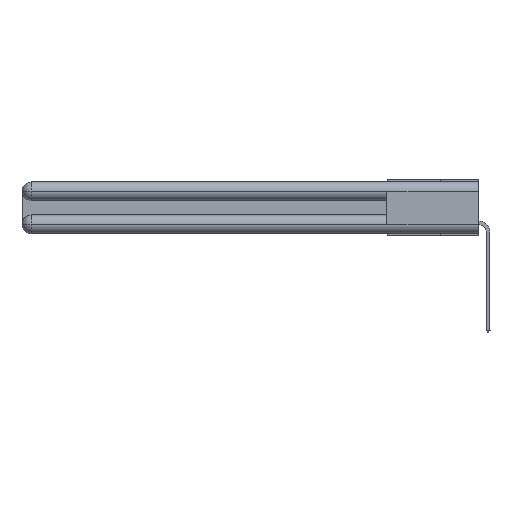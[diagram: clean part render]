
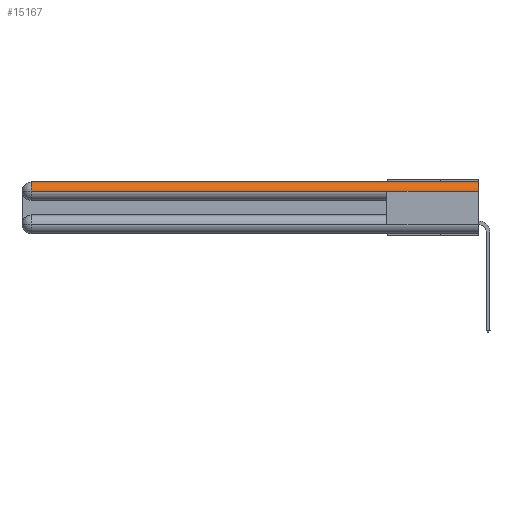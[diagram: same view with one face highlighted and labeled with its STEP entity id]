
A CAD part, left-side view. The second image highlights one B-rep face of the part: STEP entity #15167.
In plain terms, the highlighted cylindrical face has radius 1.562 mm (diameter 3.124 mm), a partial arc.
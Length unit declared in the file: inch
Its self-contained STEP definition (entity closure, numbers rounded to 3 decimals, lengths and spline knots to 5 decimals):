
#994 = CARTESIAN_POINT ( 'NONE',  ( 0., 3., -0.0615 ) ) ;
#2245 = CIRCLE ( 'NONE', #19000, 0.0615 ) ;
#2502 = VERTEX_POINT ( 'NONE', #9205 ) ;
#4608 = CARTESIAN_POINT ( 'NONE',  ( 0.0615, 0., 0. ) ) ;
#4688 = ORIENTED_EDGE ( 'NONE', *, *, #24034, .T. ) ;
#5245 = CARTESIAN_POINT ( 'NONE',  ( 0.0615, 0., -0.0615 ) ) ;
#7376 = VERTEX_POINT ( 'NONE', #23787 ) ;
#7534 = DIRECTION ( 'NONE',  ( 0., 1., 0. ) ) ;
#8774 = VECTOR ( 'NONE', #10066, 39.37008 ) ;
#9205 = CARTESIAN_POINT ( 'NONE',  ( 0., 2.94, -0.0615 ) ) ;
#9798 = LINE ( 'NONE', #21220, #12837 ) ;
#10066 = DIRECTION ( 'NONE',  ( 0., -1., 0. ) ) ;
#11555 = VERTEX_POINT ( 'NONE', #23756 ) ;
#11672 = EDGE_CURVE ( 'NONE', #27241, #13788, #25986, .T. ) ;
#11745 = DIRECTION ( 'NONE',  ( 0., 0., 1. ) ) ;
#12044 = DIRECTION ( 'NONE',  ( 0., 1., 0. ) ) ;
#12431 = VECTOR ( 'NONE', #7534, 39.37008 ) ;
#12837 = VECTOR ( 'NONE', #14884, 39.37008 ) ;
#13754 = ORIENTED_EDGE ( 'NONE', *, *, #14826, .F. ) ;
#13788 = VERTEX_POINT ( 'NONE', #4608 ) ;
#13790 = DIRECTION ( 'NONE',  ( 0., -1., 0. ) ) ;
#14197 = CARTESIAN_POINT ( 'NONE',  ( 0.0615, 0., 0. ) ) ;
#14735 = LINE ( 'NONE', #994, #12431 ) ;
#14826 = EDGE_CURVE ( 'NONE', #7376, #11555, #14735, .T. ) ;
#14884 = DIRECTION ( 'NONE',  ( 0., -1., 0. ) ) ;
#15167 = ADVANCED_FACE ( 'NONE', ( #27530 ), #21735, .T. ) ;
#16118 = DIRECTION ( 'NONE',  ( 0., -1., 0. ) ) ;
#16166 = AXIS2_PLACEMENT_3D ( 'NONE', #24703, #12044, #11745 ) ;
#17632 = EDGE_LOOP ( 'NONE', ( #18949, #4688, #21447, #13754, #26813 ) ) ;
#18093 = DIRECTION ( 'NONE',  ( 1., 0., 0. ) ) ;
#18607 = AXIS2_PLACEMENT_3D ( 'NONE', #20403, #13790, #22400 ) ;
#18905 = CIRCLE ( 'NONE', #18607, 0.0615 ) ;
#18949 = ORIENTED_EDGE ( 'NONE', *, *, #11672, .F. ) ;
#19000 = AXIS2_PLACEMENT_3D ( 'NONE', #5245, #16118, #18093 ) ;
#19574 = EDGE_CURVE ( 'NONE', #2502, #11555, #9798, .T. ) ;
#20403 = CARTESIAN_POINT ( 'NONE',  ( 0.0615, 2.94, -0.0615 ) ) ;
#21220 = CARTESIAN_POINT ( 'NONE',  ( 0., 3., -0.0615 ) ) ;
#21447 = ORIENTED_EDGE ( 'NONE', *, *, #19574, .T. ) ;
#21735 = CYLINDRICAL_SURFACE ( 'NONE', #16166, 0.0615 ) ;
#22400 = DIRECTION ( 'NONE',  ( 0., 0., 1. ) ) ;
#23756 = CARTESIAN_POINT ( 'NONE',  ( 0., 0.6, -0.0615 ) ) ;
#23787 = CARTESIAN_POINT ( 'NONE',  ( 0., 0., -0.0615 ) ) ;
#24034 = EDGE_CURVE ( 'NONE', #27241, #2502, #18905, .T. ) ;
#24703 = CARTESIAN_POINT ( 'NONE',  ( 0.0615, 0., -0.0615 ) ) ;
#25506 = CARTESIAN_POINT ( 'NONE',  ( 0.0615, 2.94, 0. ) ) ;
#25986 = LINE ( 'NONE', #14197, #8774 ) ;
#26813 = ORIENTED_EDGE ( 'NONE', *, *, #27508, .F. ) ;
#27241 = VERTEX_POINT ( 'NONE', #25506 ) ;
#27508 = EDGE_CURVE ( 'NONE', #13788, #7376, #2245, .T. ) ;
#27530 = FACE_OUTER_BOUND ( 'NONE', #17632, .T. ) ;
